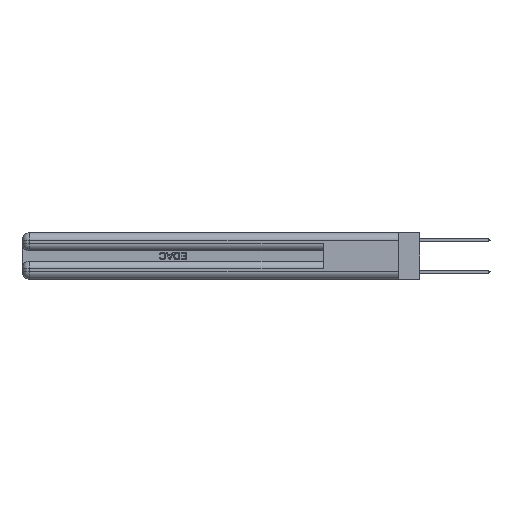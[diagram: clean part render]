
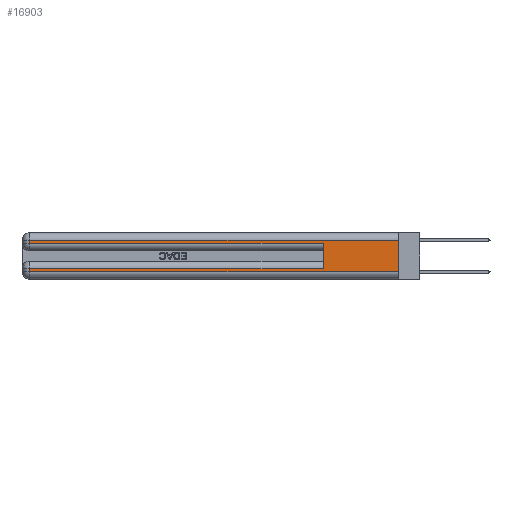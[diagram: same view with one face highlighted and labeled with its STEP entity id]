
A CAD part, left-side view. The second image highlights one B-rep face of the part: STEP entity #16903.
In plain terms, the highlighted planar face has unit normal (-1, 0, 0).
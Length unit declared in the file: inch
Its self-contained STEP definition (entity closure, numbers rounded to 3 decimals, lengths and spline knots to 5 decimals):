
#1298 = EDGE_CURVE ( 'NONE', #27756, #18086, #17618, .T. ) ;
#2334 = LINE ( 'NONE', #17512, #18913 ) ;
#2528 = VECTOR ( 'NONE', #28018, 39.37008 ) ;
#2974 = CARTESIAN_POINT ( 'NONE',  ( 0., 2.94, 0.37 ) ) ;
#3467 = DIRECTION ( 'NONE',  ( 0., 0., -1. ) ) ;
#4595 = VERTEX_POINT ( 'NONE', #5144 ) ;
#4980 = ORIENTED_EDGE ( 'NONE', *, *, #6964, .T. ) ;
#5144 = CARTESIAN_POINT ( 'NONE',  ( 0., 0.6, 0.085 ) ) ;
#6342 = LINE ( 'NONE', #27159, #7049 ) ;
#6365 = FACE_OUTER_BOUND ( 'NONE', #32274, .T. ) ;
#6677 = DIRECTION ( 'NONE',  ( 0., 0., 1. ) ) ;
#6964 = EDGE_CURVE ( 'NONE', #15045, #13062, #2334, .T. ) ;
#7049 = VECTOR ( 'NONE', #6677, 39.37008 ) ;
#7105 = CARTESIAN_POINT ( 'NONE',  ( 0., 2.94, 0.31 ) ) ;
#7788 = EDGE_CURVE ( 'NONE', #4595, #32381, #10237, .T. ) ;
#8264 = ORIENTED_EDGE ( 'NONE', *, *, #11095, .F. ) ;
#10237 = LINE ( 'NONE', #31380, #26585 ) ;
#10763 = EDGE_CURVE ( 'NONE', #13062, #15449, #28208, .T. ) ;
#11095 = EDGE_CURVE ( 'NONE', #4595, #15449, #6342, .T. ) ;
#11665 = PLANE ( 'NONE',  #13937 ) ;
#12426 = CARTESIAN_POINT ( 'NONE',  ( 0., 2.94, 0.06 ) ) ;
#13062 = VERTEX_POINT ( 'NONE', #18565 ) ;
#13937 = AXIS2_PLACEMENT_3D ( 'NONE', #14389, #24437, #3467 ) ;
#14264 = CARTESIAN_POINT ( 'NONE',  ( 0., 0., 0.37 ) ) ;
#14389 = CARTESIAN_POINT ( 'NONE',  ( 0., 0., 0.37 ) ) ;
#14455 = CARTESIAN_POINT ( 'NONE',  ( 0., 0., 0.31 ) ) ;
#14844 = ORIENTED_EDGE ( 'NONE', *, *, #10763, .T. ) ;
#14923 = EDGE_CURVE ( 'NONE', #32390, #15045, #19554, .T. ) ;
#15045 = VERTEX_POINT ( 'NONE', #7105 ) ;
#15245 = DIRECTION ( 'NONE',  ( 0., -1., 0. ) ) ;
#15449 = VERTEX_POINT ( 'NONE', #20021 ) ;
#16555 = EDGE_CURVE ( 'NONE', #32390, #18086, #32688, .T. ) ;
#16903 = ADVANCED_FACE ( 'NONE', ( #6365 ), #11665, .F. ) ;
#16976 = DIRECTION ( 'NONE',  ( 0., 0., -1. ) ) ;
#17374 = CARTESIAN_POINT ( 'NONE',  ( 0., 2.94, 0.085 ) ) ;
#17377 = VECTOR ( 'NONE', #15245, 39.37008 ) ;
#17512 = CARTESIAN_POINT ( 'NONE',  ( 0., 2.94, 0.37 ) ) ;
#17618 = LINE ( 'NONE', #27855, #2528 ) ;
#18086 = VERTEX_POINT ( 'NONE', #31650 ) ;
#18565 = CARTESIAN_POINT ( 'NONE',  ( 0., 2.94, 0.285 ) ) ;
#18913 = VECTOR ( 'NONE', #28435, 39.37008 ) ;
#19222 = DIRECTION ( 'NONE',  ( 0., 1., 0. ) ) ;
#19554 = LINE ( 'NONE', #14455, #25185 ) ;
#20021 = CARTESIAN_POINT ( 'NONE',  ( 0., 0.6, 0.285 ) ) ;
#21222 = DIRECTION ( 'NONE',  ( 0., 0., -1. ) ) ;
#22788 = EDGE_CURVE ( 'NONE', #32381, #27756, #26176, .T. ) ;
#23168 = ORIENTED_EDGE ( 'NONE', *, *, #1298, .T. ) ;
#24437 = DIRECTION ( 'NONE',  ( 1., 0., 0. ) ) ;
#24683 = VECTOR ( 'NONE', #21222, 39.37008 ) ;
#24806 = ORIENTED_EDGE ( 'NONE', *, *, #14923, .T. ) ;
#25185 = VECTOR ( 'NONE', #19222, 39.37008 ) ;
#26066 = DIRECTION ( 'NONE',  ( 0., 1., 0. ) ) ;
#26176 = LINE ( 'NONE', #2974, #24683 ) ;
#26585 = VECTOR ( 'NONE', #26066, 39.37008 ) ;
#27159 = CARTESIAN_POINT ( 'NONE',  ( 0., 0.6, 0.145 ) ) ;
#27756 = VERTEX_POINT ( 'NONE', #12426 ) ;
#27855 = CARTESIAN_POINT ( 'NONE',  ( 0., 0., 0.06 ) ) ;
#28018 = DIRECTION ( 'NONE',  ( 0., -1., 0. ) ) ;
#28208 = LINE ( 'NONE', #30771, #17377 ) ;
#28435 = DIRECTION ( 'NONE',  ( 0., 0., -1. ) ) ;
#29192 = ORIENTED_EDGE ( 'NONE', *, *, #16555, .F. ) ;
#29312 = ORIENTED_EDGE ( 'NONE', *, *, #22788, .T. ) ;
#30771 = CARTESIAN_POINT ( 'NONE',  ( 0., 0., 0.285 ) ) ;
#30834 = ORIENTED_EDGE ( 'NONE', *, *, #7788, .T. ) ;
#31380 = CARTESIAN_POINT ( 'NONE',  ( 0., 0., 0.085 ) ) ;
#31650 = CARTESIAN_POINT ( 'NONE',  ( 0., 0., 0.06 ) ) ;
#32274 = EDGE_LOOP ( 'NONE', ( #29192, #24806, #4980, #14844, #8264, #30834, #29312, #23168 ) ) ;
#32381 = VERTEX_POINT ( 'NONE', #17374 ) ;
#32390 = VERTEX_POINT ( 'NONE', #32916 ) ;
#32688 = LINE ( 'NONE', #14264, #32905 ) ;
#32905 = VECTOR ( 'NONE', #16976, 39.37008 ) ;
#32916 = CARTESIAN_POINT ( 'NONE',  ( 0., 0., 0.31 ) ) ;
